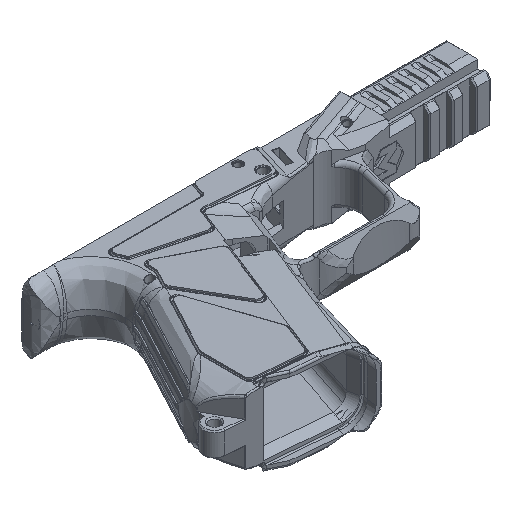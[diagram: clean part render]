
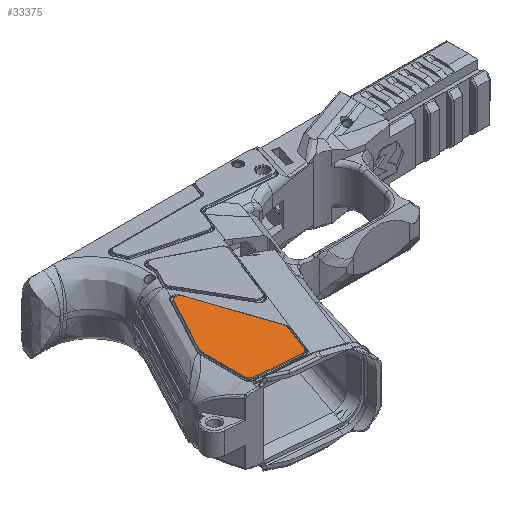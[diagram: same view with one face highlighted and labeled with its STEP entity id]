
A CAD part, isometric view. The second image highlights one B-rep face of the part: STEP entity #33375.
In plain terms, the highlighted planar face has unit normal (0, 0, 1).
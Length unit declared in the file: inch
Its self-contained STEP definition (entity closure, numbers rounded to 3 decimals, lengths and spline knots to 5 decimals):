
#310 = CARTESIAN_POINT ( 'NONE',  ( 0.62348, -1.64524, 0.58693 ) ) ;
#378 = EDGE_LOOP ( 'NONE', ( #70941, #23378, #36599, #48805, #41863, #47720, #66408, #13413, #25153, #10957, #78680 ) ) ;
#1030 = DIRECTION ( 'NONE',  ( 1., 0., 0. ) ) ;
#3214 = LINE ( 'NONE', #8868, #43922 ) ;
#3270 = DIRECTION ( 'NONE',  ( 0., 0., 1. ) ) ;
#4046 = CARTESIAN_POINT ( 'NONE',  ( 0.93659, -3.48373, 0.58693 ) ) ;
#4870 = VERTEX_POINT ( 'NONE', #310 ) ;
#4985 = VERTEX_POINT ( 'NONE', #40149 ) ;
#5049 = DIRECTION ( 'NONE',  ( 0., 0., 1. ) ) ;
#7642 = EDGE_CURVE ( 'NONE', #77946, #9644, #53643, .T. ) ;
#8868 = CARTESIAN_POINT ( 'NONE',  ( 0.92714, -1.07414, 0.58693 ) ) ;
#9644 = VERTEX_POINT ( 'NONE', #35023 ) ;
#9656 = CARTESIAN_POINT ( 'NONE',  ( 1.01814, -3.43336, 0.58693 ) ) ;
#9668 = DIRECTION ( 'NONE',  ( -0.469, -0.883, 0. ) ) ;
#10665 = AXIS2_PLACEMENT_3D ( 'NONE', #74289, #5049, #79145 ) ;
#10957 = ORIENTED_EDGE ( 'NONE', *, *, #35217, .T. ) ;
#11784 = DIRECTION ( 'NONE',  ( 1., 0., 0. ) ) ;
#12049 = VERTEX_POINT ( 'NONE', #16229 ) ;
#12728 = DIRECTION ( 'NONE',  ( 0., 0., 1. ) ) ;
#13347 = AXIS2_PLACEMENT_3D ( 'NONE', #54708, #78492, #79292 ) ;
#13413 = ORIENTED_EDGE ( 'NONE', *, *, #40553, .T. ) ;
#13491 = LINE ( 'NONE', #25974, #65777 ) ;
#14703 = DIRECTION ( 'NONE',  ( 0.367, 0.93, 0. ) ) ;
#16042 = CARTESIAN_POINT ( 'NONE',  ( 0.82976, -1.83457, 0.58693 ) ) ;
#16229 = CARTESIAN_POINT ( 'NONE',  ( 1.2021, -2.95116, 0.58693 ) ) ;
#16852 = LINE ( 'NONE', #53105, #68664 ) ;
#17139 = PLANE ( 'NONE',  #10665 ) ;
#18482 = VECTOR ( 'NONE', #22860, 39.37008 ) ;
#18774 = CARTESIAN_POINT ( 'NONE',  ( 0.19818, -3.3375, 0.58693 ) ) ;
#20812 = EDGE_CURVE ( 'NONE', #52222, #37831, #13491, .T. ) ;
#22383 = CIRCLE ( 'NONE', #13347, 0.08 ) ;
#22860 = DIRECTION ( 'NONE',  ( -0.32, 0.948, 0. ) ) ;
#23378 = ORIENTED_EDGE ( 'NONE', *, *, #35489, .T. ) ;
#24225 = LINE ( 'NONE', #42343, #42896 ) ;
#25153 = ORIENTED_EDGE ( 'NONE', *, *, #64393, .T. ) ;
#25974 = CARTESIAN_POINT ( 'NONE',  ( 0.9962, -3.48905, 0.58693 ) ) ;
#26241 = DIRECTION ( 'NONE',  ( 1., 0., 0. ) ) ;
#28874 = CIRCLE ( 'NONE', #76488, 0.08 ) ;
#29025 = DIRECTION ( 'NONE',  ( 1., 0., 0. ) ) ;
#29758 = VERTEX_POINT ( 'NONE', #45147 ) ;
#29860 = DIRECTION ( 'NONE',  ( 0.996, -0.089, 0. ) ) ;
#30426 = CARTESIAN_POINT ( 'NONE',  ( 0.69412, -1.68279, 0.58693 ) ) ;
#32464 = EDGE_CURVE ( 'NONE', #57024, #52222, #43061, .T. ) ;
#33375 = ADVANCED_FACE ( 'NONE', ( #46572 ), #17139, .T. ) ;
#34060 = EDGE_CURVE ( 'NONE', #62940, #4870, #37654, .T. ) ;
#34735 = EDGE_CURVE ( 'NONE', #29758, #62940, #47816, .T. ) ;
#35023 = CARTESIAN_POINT ( 'NONE',  ( 0.11818, -2.61552, 0.58693 ) ) ;
#35217 = EDGE_CURVE ( 'NONE', #4985, #57024, #24225, .T. ) ;
#35489 = EDGE_CURVE ( 'NONE', #37831, #12049, #22383, .T. ) ;
#36599 = ORIENTED_EDGE ( 'NONE', *, *, #79230, .T. ) ;
#37654 = CIRCLE ( 'NONE', #54374, 0.08 ) ;
#37831 = VERTEX_POINT ( 'NONE', #62019 ) ;
#37882 = AXIS2_PLACEMENT_3D ( 'NONE', #70136, #3270, #26241 ) ;
#40149 = CARTESIAN_POINT ( 'NONE',  ( 0.19107, -3.41718, 0.58693 ) ) ;
#40553 = EDGE_CURVE ( 'NONE', #9644, #70146, #16852, .T. ) ;
#41102 = DIRECTION ( 'NONE',  ( 0., 0., 1. ) ) ;
#41863 = ORIENTED_EDGE ( 'NONE', *, *, #34060, .T. ) ;
#42343 = CARTESIAN_POINT ( 'NONE',  ( 0.11818, -3.41067, 0.58693 ) ) ;
#42896 = VECTOR ( 'NONE', #29860, 39.37008 ) ;
#43061 = CIRCLE ( 'NONE', #37882, 0.08 ) ;
#43922 = VECTOR ( 'NONE', #9668, 39.37008 ) ;
#45147 = CARTESIAN_POINT ( 'NONE',  ( 1.1979, -2.92558, 0.58693 ) ) ;
#46572 = FACE_OUTER_BOUND ( 'NONE', #378, .T. ) ;
#47720 = ORIENTED_EDGE ( 'NONE', *, *, #55768, .T. ) ;
#47816 = LINE ( 'NONE', #16042, #18482 ) ;
#48805 = ORIENTED_EDGE ( 'NONE', *, *, #34735, .T. ) ;
#50576 = CARTESIAN_POINT ( 'NONE',  ( 0.12754, -2.57796, 0.58693 ) ) ;
#52004 = CARTESIAN_POINT ( 'NONE',  ( 0.19818, -2.61552, 0.58693 ) ) ;
#52222 = VERTEX_POINT ( 'NONE', #9656 ) ;
#52396 = CARTESIAN_POINT ( 'NONE',  ( 0.76992, -1.65722, 0.58693 ) ) ;
#53105 = CARTESIAN_POINT ( 'NONE',  ( 0.11818, -2.59557, 0.58693 ) ) ;
#53643 = CIRCLE ( 'NONE', #63932, 0.08 ) ;
#54374 = AXIS2_PLACEMENT_3D ( 'NONE', #30426, #67460, #73111 ) ;
#54708 = CARTESIAN_POINT ( 'NONE',  ( 1.1221, -2.95116, 0.58693 ) ) ;
#55242 = DIRECTION ( 'NONE',  ( 0., 0., 1. ) ) ;
#55768 = EDGE_CURVE ( 'NONE', #4870, #77946, #3214, .T. ) ;
#57024 = VERTEX_POINT ( 'NONE', #4046 ) ;
#58868 = CARTESIAN_POINT ( 'NONE',  ( 0.11818, -3.3375, 0.58693 ) ) ;
#61688 = CARTESIAN_POINT ( 'NONE',  ( 1.1221, -2.95116, 0.58693 ) ) ;
#62019 = CARTESIAN_POINT ( 'NONE',  ( 1.19653, -2.98048, 0.58693 ) ) ;
#62664 = CIRCLE ( 'NONE', #70487, 0.08 ) ;
#62940 = VERTEX_POINT ( 'NONE', #52396 ) ;
#63932 = AXIS2_PLACEMENT_3D ( 'NONE', #52004, #41102, #29025 ) ;
#64393 = EDGE_CURVE ( 'NONE', #70146, #4985, #28874, .T. ) ;
#65554 = DIRECTION ( 'NONE',  ( 0., -1., 0. ) ) ;
#65777 = VECTOR ( 'NONE', #14703, 39.37008 ) ;
#66408 = ORIENTED_EDGE ( 'NONE', *, *, #7642, .T. ) ;
#67460 = DIRECTION ( 'NONE',  ( 0., 0., 1. ) ) ;
#68664 = VECTOR ( 'NONE', #65554, 39.37008 ) ;
#70136 = CARTESIAN_POINT ( 'NONE',  ( 0.9437, -3.40404, 0.58693 ) ) ;
#70146 = VERTEX_POINT ( 'NONE', #58868 ) ;
#70487 = AXIS2_PLACEMENT_3D ( 'NONE', #61688, #55242, #11784 ) ;
#70941 = ORIENTED_EDGE ( 'NONE', *, *, #20812, .T. ) ;
#73111 = DIRECTION ( 'NONE',  ( 1., 0., 0. ) ) ;
#74289 = CARTESIAN_POINT ( 'NONE',  ( 5.22366, -0.35196, 0.58693 ) ) ;
#76488 = AXIS2_PLACEMENT_3D ( 'NONE', #18774, #12728, #1030 ) ;
#77946 = VERTEX_POINT ( 'NONE', #50576 ) ;
#78492 = DIRECTION ( 'NONE',  ( 0., 0., 1. ) ) ;
#78680 = ORIENTED_EDGE ( 'NONE', *, *, #32464, .T. ) ;
#79145 = DIRECTION ( 'NONE',  ( 1., 0., 0. ) ) ;
#79230 = EDGE_CURVE ( 'NONE', #12049, #29758, #62664, .T. ) ;
#79292 = DIRECTION ( 'NONE',  ( 1., 0., 0. ) ) ;
